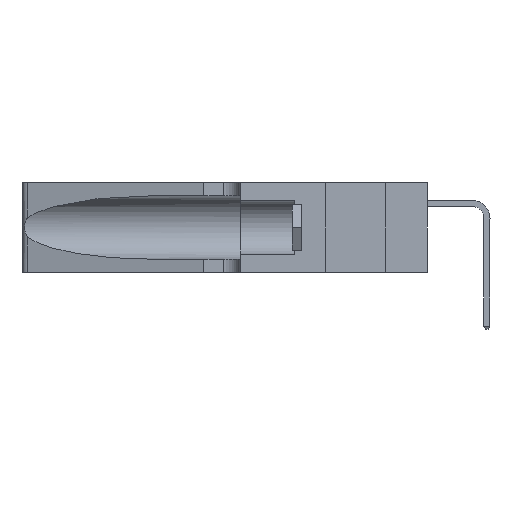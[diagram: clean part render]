
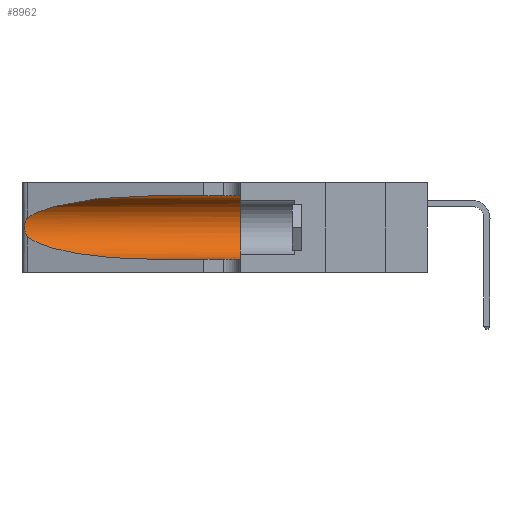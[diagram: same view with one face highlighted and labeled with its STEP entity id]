
A CAD part, left-side view. The second image highlights one B-rep face of the part: STEP entity #8962.
In plain terms, the highlighted cylindrical face has radius 3.308 mm (diameter 6.617 mm), a partial arc.
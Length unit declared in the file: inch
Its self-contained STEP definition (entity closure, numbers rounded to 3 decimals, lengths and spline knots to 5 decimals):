
#1643 = CARTESIAN_POINT ( 'NONE',  ( 0.25487, 1.22718, 0.22369 ) ) ;
#1794 = ORIENTED_EDGE ( 'NONE', *, *, #24284, .T. ) ;
#2254 = ORIENTED_EDGE ( 'NONE', *, *, #16092, .T. ) ;
#4464 = CARTESIAN_POINT ( 'NONE',  ( 0.25787, 1.23484, 0.2124 ) ) ;
#4697 = CARTESIAN_POINT ( 'NONE',  ( 0.1305, 0.72297, 0.31525 ) ) ;
#5407 = CARTESIAN_POINT ( 'NONE',  ( 0.2373, 1.15595, 0.08982 ) ) ;
#5700 = DIRECTION ( 'NONE',  ( 0., -1., 0. ) ) ;
#6501 = CIRCLE ( 'NONE', #23987, 0.13025 ) ;
#7244 = CARTESIAN_POINT ( 'NONE',  ( 0.1305, 0.35, 0.05475 ) ) ;
#7278 = EDGE_CURVE ( 'NONE', #14265, #28751, #6501, .T. ) ;
#7360 = CARTESIAN_POINT ( 'NONE',  ( 0.26018, 1.23835, 0.19895 ) ) ;
#7601 = CARTESIAN_POINT ( 'NONE',  ( 0.2373, 1.15595, 0.28018 ) ) ;
#7807 = VERTEX_POINT ( 'NONE', #12462 ) ;
#8235 = CYLINDRICAL_SURFACE ( 'NONE', #30026, 0.13025 ) ;
#8962 = ADVANCED_FACE ( 'NONE', ( #31967 ), #8235, .F. ) ;
#9490 = DIRECTION ( 'NONE',  ( 0., -1., 0. ) ) ;
#10291 = CARTESIAN_POINT ( 'NONE',  ( 0.26075, 1.23896, 0.178 ) ) ;
#11239 = CARTESIAN_POINT ( 'NONE',  ( 0.1305, 0.72297, 0.05475 ) ) ;
#11265 = EDGE_CURVE ( 'NONE', #7807, #14265, #32423, .T. ) ;
#11332 = ORIENTED_EDGE ( 'NONE', *, *, #11265, .F. ) ;
#11405 = VECTOR ( 'NONE', #5700, 39.37008 ) ;
#12381 = CARTESIAN_POINT ( 'NONE',  ( 0.1305, 1.61858, 0.185 ) ) ;
#12462 = CARTESIAN_POINT ( 'NONE',  ( 0.1305, 0.72297, 0.31525 ) ) ;
#12818 = EDGE_LOOP ( 'NONE', ( #19379, #1794, #13106, #2254, #14436, #11332 ) ) ;
#13106 = ORIENTED_EDGE ( 'NONE', *, *, #37061, .T. ) ;
#13177 = CARTESIAN_POINT ( 'NONE',  ( 0.25856, 1.23593, 0.16098 ) ) ;
#13243 = DIRECTION ( 'NONE',  ( 0., 1., 0. ) ) ;
#13616 = VERTEX_POINT ( 'NONE', #1643 ) ;
#14265 = VERTEX_POINT ( 'NONE', #22237 ) ;
#14436 = ORIENTED_EDGE ( 'NONE', *, *, #7278, .F. ) ;
#15078 = CARTESIAN_POINT ( 'NONE',  ( 0.1305, 1.61858, 0.05475 ) ) ;
#16043 = CARTESIAN_POINT ( 'NONE',  ( 0.25639, 1.23186, 0.15144 ) ) ;
#16092 = EDGE_CURVE ( 'NONE', #32286, #28751, #21377, .T. ) ;
#16423 = VERTEX_POINT ( 'NONE', #33562 ) ;
#18958 = CARTESIAN_POINT ( 'NONE',  ( 0.25487, 1.22718, 0.14631 ) ) ;
#19379 = ORIENTED_EDGE ( 'NONE', *, *, #30692, .T. ) ;
#19483 = B_SPLINE_CURVE_WITH_KNOTS ( 'NONE', 3,
 ( #32792, #33041, #21679, #4464, #24592, #7360, #27479, #10291, #30318, #13177, #33158, #16043, #35981, #18958 ),
 .UNSPECIFIED., .F., .F.,
 ( 4, 2, 2, 2, 2, 2, 4 ),
 ( 0., 0.00027, 0.00053, 0.00107, 0.0016, 0.00187, 0.00214 ),
 .UNSPECIFIED. ) ;
#20486 = VECTOR ( 'NONE', #35051, 39.37008 ) ;
#20983 =( BOUNDED_CURVE ( )  B_SPLINE_CURVE ( 3, ( #4697, #24809, #7601, #27714 ),
 .UNSPECIFIED., .F., .T. ) 
 B_SPLINE_CURVE_WITH_KNOTS ( ( 4, 4 ),
 ( 1.5708, 2.84003 ),
 .UNSPECIFIED. ) 
 CURVE ( )  GEOMETRIC_REPRESENTATION_ITEM ( )  RATIONAL_B_SPLINE_CURVE ( ( 1., 0.87, 0.87, 1. ) ) 
 REPRESENTATION_ITEM ( '' )  );
#21377 = LINE ( 'NONE', #15078, #20486 ) ;
#21679 = CARTESIAN_POINT ( 'NONE',  ( 0.25639, 1.23184, 0.21858 ) ) ;
#22237 = CARTESIAN_POINT ( 'NONE',  ( 0.1305, 0.35, 0.31525 ) ) ;
#22914 = CARTESIAN_POINT ( 'NONE',  ( 0.1305, 1.61858, 0.31525 ) ) ;
#23306 = CARTESIAN_POINT ( 'NONE',  ( 0.1305, 0.72297, 0.05475 ) ) ;
#23987 = AXIS2_PLACEMENT_3D ( 'NONE', #30391, #13243, #33226 ) ;
#24284 = EDGE_CURVE ( 'NONE', #13616, #16423, #19483, .T. ) ;
#24592 = CARTESIAN_POINT ( 'NONE',  ( 0.25854, 1.2359, 0.20912 ) ) ;
#24809 = CARTESIAN_POINT ( 'NONE',  ( 0.18966, 0.96281, 0.31525 ) ) ;
#25529 = CARTESIAN_POINT ( 'NONE',  ( 0.25487, 1.22718, 0.14631 ) ) ;
#27479 = CARTESIAN_POINT ( 'NONE',  ( 0.26075, 1.23896, 0.19203 ) ) ;
#27714 = CARTESIAN_POINT ( 'NONE',  ( 0.25487, 1.22718, 0.22369 ) ) ;
#28393 = CARTESIAN_POINT ( 'NONE',  ( 0.18966, 0.96281, 0.05475 ) ) ;
#28751 = VERTEX_POINT ( 'NONE', #7244 ) ;
#30026 = AXIS2_PLACEMENT_3D ( 'NONE', #12381, #9490, #32376 ) ;
#30318 = CARTESIAN_POINT ( 'NONE',  ( 0.26017, 1.23833, 0.17102 ) ) ;
#30391 = CARTESIAN_POINT ( 'NONE',  ( 0.1305, 0.35, 0.185 ) ) ;
#30692 = EDGE_CURVE ( 'NONE', #7807, #13616, #20983, .T. ) ;
#31967 = FACE_OUTER_BOUND ( 'NONE', #12818, .T. ) ;
#32286 = VERTEX_POINT ( 'NONE', #23306 ) ;
#32376 = DIRECTION ( 'NONE',  ( 0., 0., -1. ) ) ;
#32423 = LINE ( 'NONE', #22914, #11405 ) ;
#32792 = CARTESIAN_POINT ( 'NONE',  ( 0.25487, 1.22718, 0.22369 ) ) ;
#33041 = CARTESIAN_POINT ( 'NONE',  ( 0.25555, 1.22994, 0.2215 ) ) ;
#33158 = CARTESIAN_POINT ( 'NONE',  ( 0.25789, 1.23486, 0.15765 ) ) ;
#33226 = DIRECTION ( 'NONE',  ( 0., 0., 1. ) ) ;
#33562 = CARTESIAN_POINT ( 'NONE',  ( 0.25487, 1.22718, 0.14631 ) ) ;
#35051 = DIRECTION ( 'NONE',  ( 0., -1., 0. ) ) ;
#35981 = CARTESIAN_POINT ( 'NONE',  ( 0.25555, 1.22993, 0.14849 ) ) ;
#36215 =( BOUNDED_CURVE ( )  B_SPLINE_CURVE ( 3, ( #25529, #5407, #28393, #11239 ),
 .UNSPECIFIED., .F., .F. ) 
 B_SPLINE_CURVE_WITH_KNOTS ( ( 4, 4 ),
 ( 3.44316, 4.71239 ),
 .UNSPECIFIED. ) 
 CURVE ( )  GEOMETRIC_REPRESENTATION_ITEM ( )  RATIONAL_B_SPLINE_CURVE ( ( 1., 0.87, 0.87, 1. ) ) 
 REPRESENTATION_ITEM ( '' )  );
#37061 = EDGE_CURVE ( 'NONE', #16423, #32286, #36215, .T. ) ;
